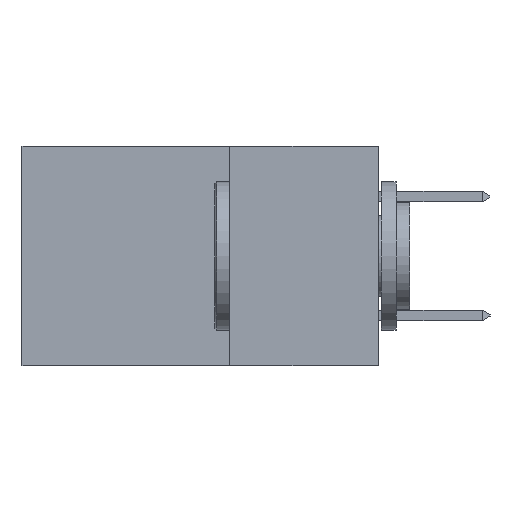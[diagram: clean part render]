
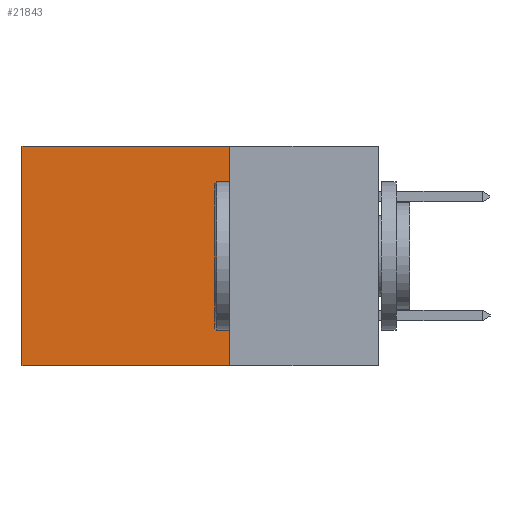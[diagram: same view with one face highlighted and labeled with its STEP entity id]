
A CAD part, left-side view. The second image highlights one B-rep face of the part: STEP entity #21843.
In plain terms, the highlighted planar face has unit normal (-1, 0, 0).
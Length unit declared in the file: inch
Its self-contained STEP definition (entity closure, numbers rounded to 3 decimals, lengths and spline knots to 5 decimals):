
#519 = VECTOR ( 'NONE', #14485, 39.37008 ) ;
#1628 = VERTEX_POINT ( 'NONE', #21844 ) ;
#3093 = FACE_OUTER_BOUND ( 'NONE', #12155, .T. ) ;
#3291 = VECTOR ( 'NONE', #24737, 39.37008 ) ;
#3610 = CARTESIAN_POINT ( 'NONE',  ( 0.2615, 0.25, -0.37 ) ) ;
#3612 = CARTESIAN_POINT ( 'NONE',  ( 0.2615, 0.6, -0.37 ) ) ;
#3966 = EDGE_CURVE ( 'NONE', #1628, #14246, #4484, .T. ) ;
#4484 = LINE ( 'NONE', #20544, #25808 ) ;
#4929 = DIRECTION ( 'NONE',  ( 0., 1., 0. ) ) ;
#5701 = DIRECTION ( 'NONE',  ( 1., 0., 0. ) ) ;
#6281 = EDGE_CURVE ( 'NONE', #1628, #18773, #10349, .T. ) ;
#7093 = LINE ( 'NONE', #21373, #12676 ) ;
#8547 = CARTESIAN_POINT ( 'NONE',  ( 0.2615, 0.25, -0.37 ) ) ;
#8860 = ORIENTED_EDGE ( 'NONE', *, *, #6281, .T. ) ;
#9597 = EDGE_CURVE ( 'NONE', #18773, #13279, #15033, .T. ) ;
#10349 = LINE ( 'NONE', #14393, #519 ) ;
#12155 = EDGE_LOOP ( 'NONE', ( #24455, #19676, #21388, #8860 ) ) ;
#12497 = CARTESIAN_POINT ( 'NONE',  ( 0.2615, 0.6, -0.37 ) ) ;
#12676 = VECTOR ( 'NONE', #4929, 39.37008 ) ;
#13279 = VERTEX_POINT ( 'NONE', #3612 ) ;
#14246 = VERTEX_POINT ( 'NONE', #8547 ) ;
#14393 = CARTESIAN_POINT ( 'NONE',  ( 0.2615, 0.25, 0. ) ) ;
#14485 = DIRECTION ( 'NONE',  ( 0., 1., 0. ) ) ;
#15033 = LINE ( 'NONE', #12497, #3291 ) ;
#15338 = CARTESIAN_POINT ( 'NONE',  ( 0.2615, 0.6, 0. ) ) ;
#16075 = PLANE ( 'NONE',  #24372 ) ;
#18773 = VERTEX_POINT ( 'NONE', #15338 ) ;
#19676 = ORIENTED_EDGE ( 'NONE', *, *, #26400, .F. ) ;
#20155 = DIRECTION ( 'NONE',  ( 0., 0., -1. ) ) ;
#20252 = DIRECTION ( 'NONE',  ( 0., 0., -1. ) ) ;
#20544 = CARTESIAN_POINT ( 'NONE',  ( 0.2615, 0.25, -0.37 ) ) ;
#21373 = CARTESIAN_POINT ( 'NONE',  ( 0.2615, 0.25, -0.37 ) ) ;
#21388 = ORIENTED_EDGE ( 'NONE', *, *, #3966, .F. ) ;
#21843 = ADVANCED_FACE ( 'NONE', ( #3093 ), #16075, .F. ) ;
#21844 = CARTESIAN_POINT ( 'NONE',  ( 0.2615, 0.25, 0. ) ) ;
#24372 = AXIS2_PLACEMENT_3D ( 'NONE', #3610, #5701, #20155 ) ;
#24455 = ORIENTED_EDGE ( 'NONE', *, *, #9597, .T. ) ;
#24737 = DIRECTION ( 'NONE',  ( 0., 0., -1. ) ) ;
#25808 = VECTOR ( 'NONE', #20252, 39.37008 ) ;
#26400 = EDGE_CURVE ( 'NONE', #14246, #13279, #7093, .T. ) ;
